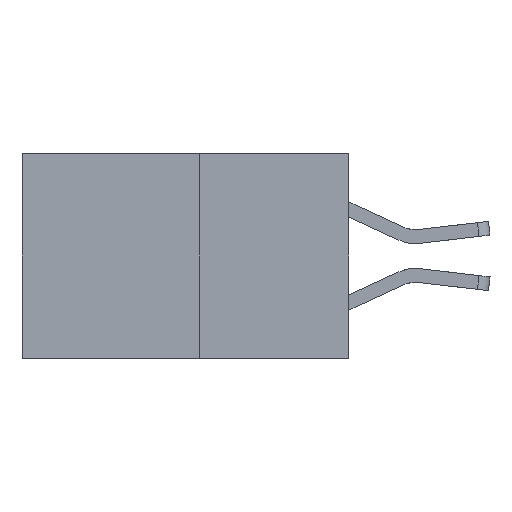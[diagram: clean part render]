
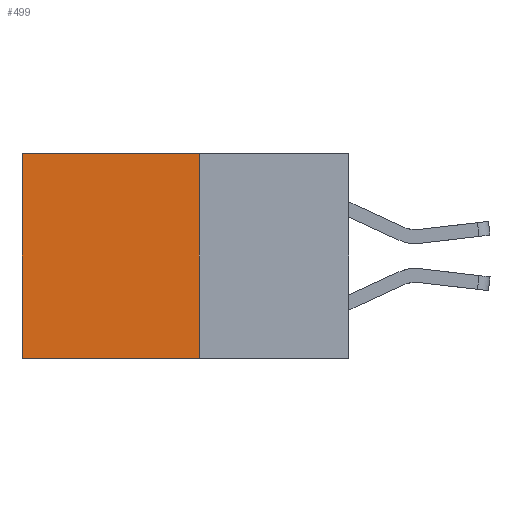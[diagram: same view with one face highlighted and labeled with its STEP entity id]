
A CAD part, left-side view. The second image highlights one B-rep face of the part: STEP entity #499.
In plain terms, the highlighted planar face has unit normal (-1, 0, 0).
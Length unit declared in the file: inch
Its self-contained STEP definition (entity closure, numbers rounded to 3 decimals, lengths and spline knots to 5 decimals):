
#183 = DIRECTION ( 'NONE',  ( 0., 0., -1. ) ) ;
#255 = LINE ( 'NONE', #4296, #2675 ) ;
#499 = ADVANCED_FACE ( 'NONE', ( #8771 ), #793, .F. ) ;
#793 = PLANE ( 'NONE',  #5532 ) ;
#860 = ORIENTED_EDGE ( 'NONE', *, *, #3486, .T. ) ;
#1507 = EDGE_LOOP ( 'NONE', ( #6386, #5744, #2049, #860 ) ) ;
#1580 = VERTEX_POINT ( 'NONE', #5675 ) ;
#2049 = ORIENTED_EDGE ( 'NONE', *, *, #2891, .F. ) ;
#2052 = CARTESIAN_POINT ( 'NONE',  ( 0.277, 0.59, 0. ) ) ;
#2054 = VERTEX_POINT ( 'NONE', #7742 ) ;
#2119 = CARTESIAN_POINT ( 'NONE',  ( 0.277, 0.27, -0.37 ) ) ;
#2675 = VECTOR ( 'NONE', #183, 39.37008 ) ;
#2891 = EDGE_CURVE ( 'NONE', #2054, #1580, #7337, .T. ) ;
#3486 = EDGE_CURVE ( 'NONE', #2054, #9616, #5051, .T. ) ;
#3487 = DIRECTION ( 'NONE',  ( 1., 0., 0. ) ) ;
#3649 = DIRECTION ( 'NONE',  ( 0., 1., 0. ) ) ;
#3661 = CARTESIAN_POINT ( 'NONE',  ( 0.277, 0.27, 0. ) ) ;
#4296 = CARTESIAN_POINT ( 'NONE',  ( 0.277, 0.59, -0.37 ) ) ;
#4526 = DIRECTION ( 'NONE',  ( 0., 0., -1. ) ) ;
#5016 = CARTESIAN_POINT ( 'NONE',  ( 0.277, 0.27, -0.37 ) ) ;
#5051 = LINE ( 'NONE', #3661, #7434 ) ;
#5075 = VECTOR ( 'NONE', #6370, 39.37008 ) ;
#5122 = CARTESIAN_POINT ( 'NONE',  ( 0.277, 0.59, -0.37 ) ) ;
#5532 = AXIS2_PLACEMENT_3D ( 'NONE', #2119, #3487, #7355 ) ;
#5654 = VERTEX_POINT ( 'NONE', #5122 ) ;
#5675 = CARTESIAN_POINT ( 'NONE',  ( 0.277, 0.27, -0.37 ) ) ;
#5744 = ORIENTED_EDGE ( 'NONE', *, *, #9598, .F. ) ;
#6370 = DIRECTION ( 'NONE',  ( 0., 1., 0. ) ) ;
#6386 = ORIENTED_EDGE ( 'NONE', *, *, #8617, .T. ) ;
#7038 = LINE ( 'NONE', #9187, #5075 ) ;
#7337 = LINE ( 'NONE', #5016, #9001 ) ;
#7355 = DIRECTION ( 'NONE',  ( 0., 0., -1. ) ) ;
#7434 = VECTOR ( 'NONE', #3649, 39.37008 ) ;
#7742 = CARTESIAN_POINT ( 'NONE',  ( 0.277, 0.27, 0. ) ) ;
#8617 = EDGE_CURVE ( 'NONE', #9616, #5654, #255, .T. ) ;
#8771 = FACE_OUTER_BOUND ( 'NONE', #1507, .T. ) ;
#9001 = VECTOR ( 'NONE', #4526, 39.37008 ) ;
#9187 = CARTESIAN_POINT ( 'NONE',  ( 0.277, 0.27, -0.37 ) ) ;
#9598 = EDGE_CURVE ( 'NONE', #1580, #5654, #7038, .T. ) ;
#9616 = VERTEX_POINT ( 'NONE', #2052 ) ;
